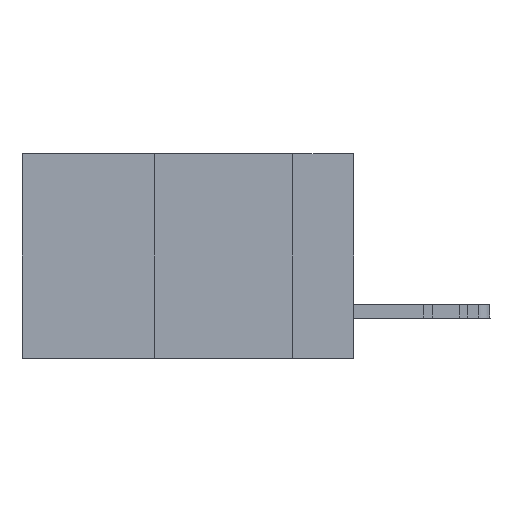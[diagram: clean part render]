
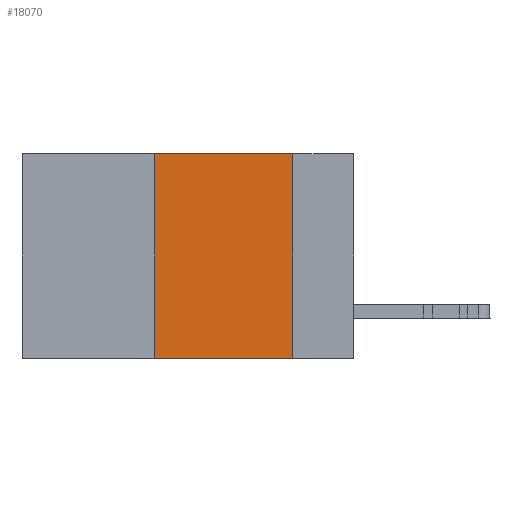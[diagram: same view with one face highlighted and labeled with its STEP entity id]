
A CAD part, left-side view. The second image highlights one B-rep face of the part: STEP entity #18070.
In plain terms, the highlighted planar face has unit normal (-1, 0, 0).
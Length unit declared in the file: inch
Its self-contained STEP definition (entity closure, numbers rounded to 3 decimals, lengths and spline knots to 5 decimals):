
#380 = LINE ( 'NONE', #28709, #18619 ) ;
#1233 = CARTESIAN_POINT ( 'NONE',  ( 0., 0.36, 0. ) ) ;
#2527 = DIRECTION ( 'NONE',  ( 0., -1., 0. ) ) ;
#4283 = ORIENTED_EDGE ( 'NONE', *, *, #36181, .F. ) ;
#4956 = VERTEX_POINT ( 'NONE', #19639 ) ;
#5025 = EDGE_CURVE ( 'NONE', #24062, #42392, #36941, .T. ) ;
#5163 = PLANE ( 'NONE',  #10149 ) ;
#8002 = EDGE_CURVE ( 'NONE', #42392, #25758, #35242, .T. ) ;
#8676 = DIRECTION ( 'NONE',  ( 0., 0., -1. ) ) ;
#8933 = DIRECTION ( 'NONE',  ( 1., 0., 0. ) ) ;
#9867 = CARTESIAN_POINT ( 'NONE',  ( 0., 0.6, -0.37 ) ) ;
#10149 = AXIS2_PLACEMENT_3D ( 'NONE', #27417, #8933, #12549 ) ;
#12549 = DIRECTION ( 'NONE',  ( 0., 0., -1. ) ) ;
#13965 = VECTOR ( 'NONE', #2527, 39.37008 ) ;
#13994 = FACE_OUTER_BOUND ( 'NONE', #42017, .T. ) ;
#17024 = CARTESIAN_POINT ( 'NONE',  ( 0., 0.11, -0.37 ) ) ;
#18070 = ADVANCED_FACE ( 'NONE', ( #13994 ), #5163, .F. ) ;
#18619 = VECTOR ( 'NONE', #24811, 39.37008 ) ;
#19639 = CARTESIAN_POINT ( 'NONE',  ( 0., 0.36, -0.37 ) ) ;
#24062 = VERTEX_POINT ( 'NONE', #1233 ) ;
#24811 = DIRECTION ( 'NONE',  ( 0., 0., 1. ) ) ;
#25330 = VECTOR ( 'NONE', #41817, 39.37008 ) ;
#25452 = VECTOR ( 'NONE', #8676, 39.37008 ) ;
#25758 = VERTEX_POINT ( 'NONE', #17024 ) ;
#27417 = CARTESIAN_POINT ( 'NONE',  ( 0., 0.6, 0. ) ) ;
#28709 = CARTESIAN_POINT ( 'NONE',  ( 0., 0.36, 0. ) ) ;
#32667 = LINE ( 'NONE', #9867, #13965 ) ;
#35183 = EDGE_CURVE ( 'NONE', #4956, #25758, #32667, .T. ) ;
#35242 = LINE ( 'NONE', #37232, #25452 ) ;
#35621 = CARTESIAN_POINT ( 'NONE',  ( 0., 0.11, 0. ) ) ;
#36181 = EDGE_CURVE ( 'NONE', #4956, #24062, #380, .T. ) ;
#36941 = LINE ( 'NONE', #42822, #25330 ) ;
#37232 = CARTESIAN_POINT ( 'NONE',  ( 0., 0.11, 0. ) ) ;
#38921 = ORIENTED_EDGE ( 'NONE', *, *, #8002, .F. ) ;
#41690 = ORIENTED_EDGE ( 'NONE', *, *, #5025, .F. ) ;
#41817 = DIRECTION ( 'NONE',  ( 0., -1., 0. ) ) ;
#42017 = EDGE_LOOP ( 'NONE', ( #38921, #41690, #4283, #45942 ) ) ;
#42392 = VERTEX_POINT ( 'NONE', #35621 ) ;
#42822 = CARTESIAN_POINT ( 'NONE',  ( 0., 0.6, 0. ) ) ;
#45942 = ORIENTED_EDGE ( 'NONE', *, *, #35183, .T. ) ;
